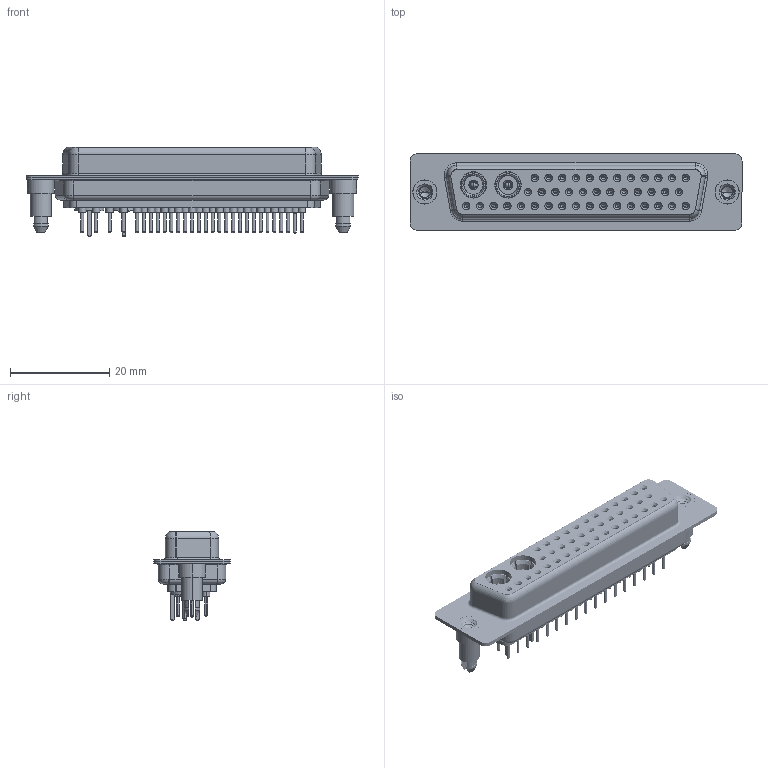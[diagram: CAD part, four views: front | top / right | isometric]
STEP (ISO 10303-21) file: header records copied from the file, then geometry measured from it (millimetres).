
FILE_DESCRIPTION (( 'STEP AP203' ), '1' );
FILE_NAME ('628-43W2624-5N5.STEP', '2019-06-26T21:19:32', ( '' ), ( '' ), 'SwSTEP 2.0', 'SolidWorks 2016', '' );
FILE_SCHEMA (( 'CONFIG_CONTROL_DESIGN' ));
Length unit declared in the file: millimetre
Products named in the file (13): 628Combo Contact Row 3_24; 628Combo Contact Row 1_24; 628-43W2624-5N5; 628Combo Shell Rear_50 Contacts; 628Combo Contact Row 2_24; Co-Ax Plug Assy_St; Pin_Str; 628Combo Threaded Boardlock_5; 628Combo Shell Front_50 Contacts; Insulator Pin_Straight PC Tail; Co-Ax Plug_Straight PC Tail; Locking Collar; 628Combo Housing_43W2
Assembly tree (52 placements, depth 3):
  628-43W2624-5N5
    628Combo Housing_43W2
    628Combo Shell Front_50 Contacts
    628Combo Shell Rear_50 Contacts
    628Combo Threaded Boardlock_5  x2
    628Combo Contact Row 1_24  x12
    628Combo Contact Row 2_24  x12
    628Combo Contact Row 3_24  x17
    Co-Ax Plug Assy_St  x2
      Co-Ax Plug_Straight PC Tail
      Insulator Pin_Straight PC Tail
      Pin_Str
      Locking Collar
Bounding box: 67 x 15.4 x 18.15 mm (x, y, z)
Volume: 7063.9 mm3; surface area: 15314.3 mm2
Topology: 54 solids, 54 shells, 2838 faces, 6593 edges, 4058 vertices
Faces by surface type: cylinder 1038, plane 812, torus 639, cone 331, bspline 10, sphere 8
Entity records: 34839 total; most frequent: CARTESIAN_POINT 7171, DIRECTION 5846, ORIENTED_EDGE 4830, AXIS2_PLACEMENT_3D 2464, EDGE_CURVE 2415, VERTEX_POINT 1535, CIRCLE 1351, EDGE_LOOP 1324
